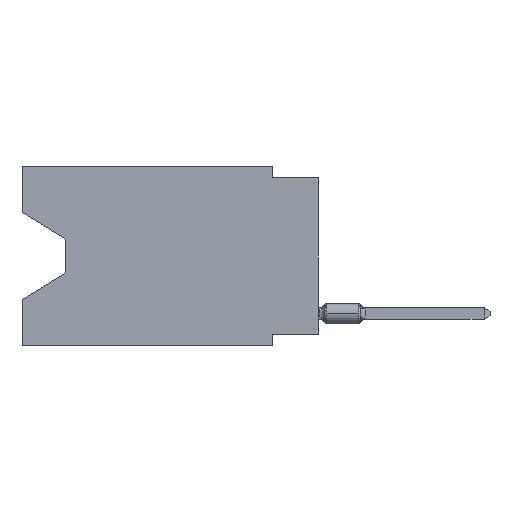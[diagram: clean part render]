
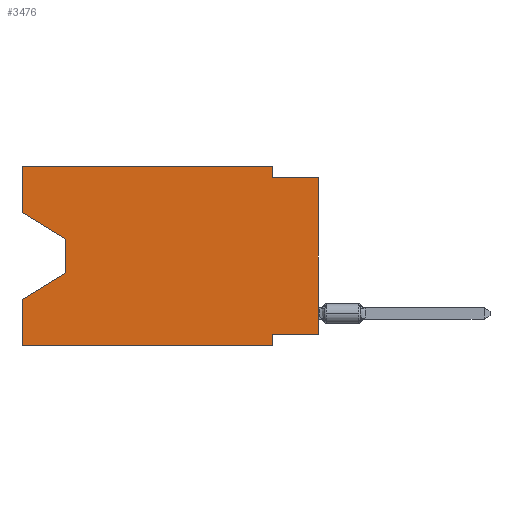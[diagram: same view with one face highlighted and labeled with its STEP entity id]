
A CAD part, left-side view. The second image highlights one B-rep face of the part: STEP entity #3476.
In plain terms, the highlighted planar face has unit normal (-1, 0, 0).
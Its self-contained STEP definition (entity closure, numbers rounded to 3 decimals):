
#16 = LINE ( 'NONE', #3380, #1217 ) ;
#271 = EDGE_CURVE ( 'NONE', #7617, #13160, #16090, .T. ) ;
#303 = DIRECTION ( 'NONE',  ( 0., 1., 0. ) ) ;
#497 = ORIENTED_EDGE ( 'NONE', *, *, #12654, .T. ) ;
#523 = VECTOR ( 'NONE', #15396, 1000. ) ;
#910 = VECTOR ( 'NONE', #17451, 1000. ) ;
#966 = CARTESIAN_POINT ( 'NONE',  ( 0., 16.383, 0. ) ) ;
#1217 = VECTOR ( 'NONE', #303, 1000. ) ;
#1241 = VERTEX_POINT ( 'NONE', #11429 ) ;
#1309 = VERTEX_POINT ( 'NONE', #9132 ) ;
#1458 = VECTOR ( 'NONE', #5962, 1000. ) ;
#1557 = EDGE_CURVE ( 'NONE', #1309, #7302, #11202, .T. ) ;
#2099 = DIRECTION ( 'NONE',  ( 0., -0.855, -0.519 ) ) ;
#2130 = CARTESIAN_POINT ( 'NONE',  ( 0., 16.383, -7.36 ) ) ;
#2268 = VECTOR ( 'NONE', #2099, 1000. ) ;
#2387 = EDGE_CURVE ( 'NONE', #13807, #5778, #16705, .T. ) ;
#2587 = ORIENTED_EDGE ( 'NONE', *, *, #1557, .F. ) ;
#2788 = CARTESIAN_POINT ( 'NONE',  ( 0., 16.383, 0. ) ) ;
#3204 = EDGE_CURVE ( 'NONE', #1241, #13160, #3666, .T. ) ;
#3380 = CARTESIAN_POINT ( 'NONE',  ( 0., 0., -9.271 ) ) ;
#3415 = LINE ( 'NONE', #9480, #910 ) ;
#3476 = ADVANCED_FACE ( 'NONE', ( #12221 ), #13621, .F. ) ;
#3511 = ORIENTED_EDGE ( 'NONE', *, *, #2387, .F. ) ;
#3666 = LINE ( 'NONE', #14026, #16345 ) ;
#4372 = LINE ( 'NONE', #4568, #4894 ) ;
#4568 = CARTESIAN_POINT ( 'NONE',  ( 0., 16.383, -9.906 ) ) ;
#4594 = VECTOR ( 'NONE', #14204, 1000. ) ;
#4768 = CARTESIAN_POINT ( 'NONE',  ( 0., 16.383, 0. ) ) ;
#4894 = VECTOR ( 'NONE', #19500, 1000. ) ;
#5376 = CARTESIAN_POINT ( 'NONE',  ( 0., 16.383, -2.546 ) ) ;
#5534 = EDGE_CURVE ( 'NONE', #7043, #1241, #7623, .T. ) ;
#5778 = VERTEX_POINT ( 'NONE', #13198 ) ;
#5962 = DIRECTION ( 'NONE',  ( 0., 0., 1. ) ) ;
#6375 = ORIENTED_EDGE ( 'NONE', *, *, #7810, .T. ) ;
#6432 = ORIENTED_EDGE ( 'NONE', *, *, #18156, .F. ) ;
#6551 = CARTESIAN_POINT ( 'NONE',  ( 0., 13.97, -5.893 ) ) ;
#6613 = CARTESIAN_POINT ( 'NONE',  ( 0., 0., -9.271 ) ) ;
#7012 = CARTESIAN_POINT ( 'NONE',  ( 0., 0., 0. ) ) ;
#7043 = VERTEX_POINT ( 'NONE', #7940 ) ;
#7161 = LINE ( 'NONE', #2788, #1458 ) ;
#7275 = VERTEX_POINT ( 'NONE', #9197 ) ;
#7302 = VERTEX_POINT ( 'NONE', #2130 ) ;
#7376 = DIRECTION ( 'NONE',  ( 0., -1., 0. ) ) ;
#7617 = VERTEX_POINT ( 'NONE', #6613 ) ;
#7623 = LINE ( 'NONE', #10800, #523 ) ;
#7810 = EDGE_CURVE ( 'NONE', #13036, #7302, #13114, .T. ) ;
#7940 = CARTESIAN_POINT ( 'NONE',  ( 0., 2.54, 0. ) ) ;
#8927 = DIRECTION ( 'NONE',  ( 0., 0., -1. ) ) ;
#9033 = EDGE_CURVE ( 'NONE', #11993, #7275, #12845, .T. ) ;
#9129 = CARTESIAN_POINT ( 'NONE',  ( 0., 16.383, 0. ) ) ;
#9132 = CARTESIAN_POINT ( 'NONE',  ( 0., 16.383, -9.906 ) ) ;
#9197 = CARTESIAN_POINT ( 'NONE',  ( 0., 13.97, -4.013 ) ) ;
#9480 = CARTESIAN_POINT ( 'NONE',  ( 0., 13.97, -4.013 ) ) ;
#9936 = CARTESIAN_POINT ( 'NONE',  ( 0., 0., -0.635 ) ) ;
#10151 = DIRECTION ( 'NONE',  ( 1., 0., 0. ) ) ;
#10274 = CARTESIAN_POINT ( 'NONE',  ( 0., 16.383, 0. ) ) ;
#10800 = CARTESIAN_POINT ( 'NONE',  ( 0., 2.54, 0. ) ) ;
#10828 = EDGE_CURVE ( 'NONE', #17182, #7043, #14963, .T. ) ;
#11041 = ORIENTED_EDGE ( 'NONE', *, *, #16458, .T. ) ;
#11199 = DIRECTION ( 'NONE',  ( 0., 0., 1. ) ) ;
#11202 = LINE ( 'NONE', #966, #4594 ) ;
#11429 = CARTESIAN_POINT ( 'NONE',  ( 0., 2.54, -0.635 ) ) ;
#11620 = ORIENTED_EDGE ( 'NONE', *, *, #9033, .T. ) ;
#11623 = DIRECTION ( 'NONE',  ( 0., 0.855, -0.519 ) ) ;
#11993 = VERTEX_POINT ( 'NONE', #18650 ) ;
#12221 = FACE_OUTER_BOUND ( 'NONE', #12569, .T. ) ;
#12240 = VECTOR ( 'NONE', #8927, 1000. ) ;
#12363 = ORIENTED_EDGE ( 'NONE', *, *, #13996, .F. ) ;
#12569 = EDGE_LOOP ( 'NONE', ( #11620, #11041, #6375, #2587, #497, #3511, #6432, #18209, #18172, #18739, #12940, #12363 ) ) ;
#12654 = EDGE_CURVE ( 'NONE', #1309, #5778, #4372, .T. ) ;
#12845 = LINE ( 'NONE', #5376, #2268 ) ;
#12940 = ORIENTED_EDGE ( 'NONE', *, *, #10828, .F. ) ;
#13036 = VERTEX_POINT ( 'NONE', #6551 ) ;
#13114 = LINE ( 'NONE', #19181, #14144 ) ;
#13160 = VERTEX_POINT ( 'NONE', #9936 ) ;
#13198 = CARTESIAN_POINT ( 'NONE',  ( 0., 2.54, -9.906 ) ) ;
#13524 = CARTESIAN_POINT ( 'NONE',  ( 0., 2.54, -9.906 ) ) ;
#13621 = PLANE ( 'NONE',  #15095 ) ;
#13750 = CARTESIAN_POINT ( 'NONE',  ( 0., 2.54, -9.271 ) ) ;
#13807 = VERTEX_POINT ( 'NONE', #13750 ) ;
#13996 = EDGE_CURVE ( 'NONE', #11993, #17182, #7161, .T. ) ;
#14026 = CARTESIAN_POINT ( 'NONE',  ( 0., 0., -0.635 ) ) ;
#14144 = VECTOR ( 'NONE', #11623, 1000. ) ;
#14204 = DIRECTION ( 'NONE',  ( 0., 0., 1. ) ) ;
#14963 = LINE ( 'NONE', #10274, #17529 ) ;
#15095 = AXIS2_PLACEMENT_3D ( 'NONE', #9129, #10151, #17901 ) ;
#15396 = DIRECTION ( 'NONE',  ( 0., 0., -1. ) ) ;
#15525 = DIRECTION ( 'NONE',  ( 0., -1., 0. ) ) ;
#16090 = LINE ( 'NONE', #7012, #19177 ) ;
#16345 = VECTOR ( 'NONE', #15525, 1000. ) ;
#16458 = EDGE_CURVE ( 'NONE', #7275, #13036, #3415, .T. ) ;
#16705 = LINE ( 'NONE', #13524, #12240 ) ;
#17182 = VERTEX_POINT ( 'NONE', #4768 ) ;
#17451 = DIRECTION ( 'NONE',  ( 0., 0., -1. ) ) ;
#17529 = VECTOR ( 'NONE', #7376, 1000. ) ;
#17901 = DIRECTION ( 'NONE',  ( 0., 0., -1. ) ) ;
#18156 = EDGE_CURVE ( 'NONE', #7617, #13807, #16, .T. ) ;
#18172 = ORIENTED_EDGE ( 'NONE', *, *, #3204, .F. ) ;
#18209 = ORIENTED_EDGE ( 'NONE', *, *, #271, .T. ) ;
#18650 = CARTESIAN_POINT ( 'NONE',  ( 0., 16.383, -2.546 ) ) ;
#18739 = ORIENTED_EDGE ( 'NONE', *, *, #5534, .F. ) ;
#19177 = VECTOR ( 'NONE', #11199, 1000. ) ;
#19181 = CARTESIAN_POINT ( 'NONE',  ( 0., 13.97, -5.893 ) ) ;
#19500 = DIRECTION ( 'NONE',  ( 0., -1., 0. ) ) ;
